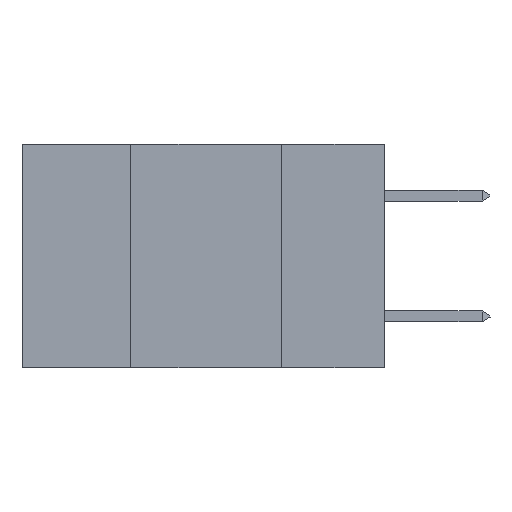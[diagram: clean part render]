
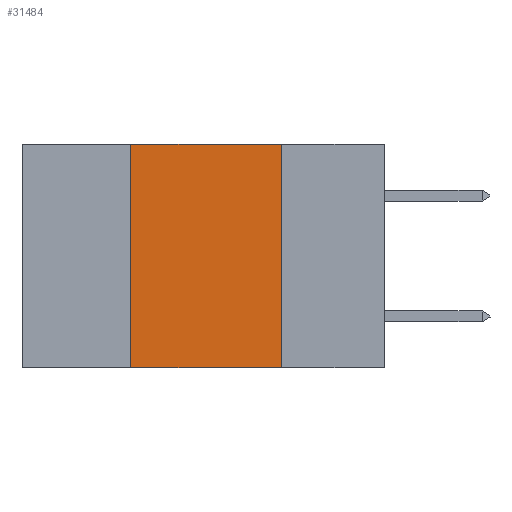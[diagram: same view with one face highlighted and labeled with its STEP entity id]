
A CAD part, left-side view. The second image highlights one B-rep face of the part: STEP entity #31484.
In plain terms, the highlighted planar face has unit normal (-1, 0, 0).
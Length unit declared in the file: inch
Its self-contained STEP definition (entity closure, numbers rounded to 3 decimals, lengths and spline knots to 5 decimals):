
#543 = FACE_OUTER_BOUND ( 'NONE', #5892, .T. ) ;
#1035 = CARTESIAN_POINT ( 'NONE',  ( 0., 0.6, -0.37 ) ) ;
#2490 = CARTESIAN_POINT ( 'NONE',  ( 0., 0.17, -0.37 ) ) ;
#3520 = ORIENTED_EDGE ( 'NONE', *, *, #5733, .F. ) ;
#5733 = EDGE_CURVE ( 'NONE', #18962, #36356, #24256, .T. ) ;
#5892 = EDGE_LOOP ( 'NONE', ( #11558, #26193, #3520, #23856 ) ) ;
#5940 = VECTOR ( 'NONE', #36584, 39.37008 ) ;
#8122 = LINE ( 'NONE', #17236, #39763 ) ;
#10659 = DIRECTION ( 'NONE',  ( 0., -1., 0. ) ) ;
#11173 = LINE ( 'NONE', #16390, #33900 ) ;
#11558 = ORIENTED_EDGE ( 'NONE', *, *, #17591, .F. ) ;
#14889 = DIRECTION ( 'NONE',  ( 1., 0., 0. ) ) ;
#16390 = CARTESIAN_POINT ( 'NONE',  ( 0., 0.17, 0. ) ) ;
#17236 = CARTESIAN_POINT ( 'NONE',  ( 0., 0.6, 0. ) ) ;
#17346 = CARTESIAN_POINT ( 'NONE',  ( 0., 0.42, 0. ) ) ;
#17591 = EDGE_CURVE ( 'NONE', #40217, #25100, #11173, .T. ) ;
#18962 = VERTEX_POINT ( 'NONE', #36440 ) ;
#19039 = CARTESIAN_POINT ( 'NONE',  ( 0., 0.42, 0. ) ) ;
#21131 = PLANE ( 'NONE',  #21215 ) ;
#21215 = AXIS2_PLACEMENT_3D ( 'NONE', #30501, #14889, #23902 ) ;
#23856 = ORIENTED_EDGE ( 'NONE', *, *, #30730, .T. ) ;
#23902 = DIRECTION ( 'NONE',  ( 0., 0., -1. ) ) ;
#24256 = LINE ( 'NONE', #17346, #5940 ) ;
#24322 = LINE ( 'NONE', #1035, #34721 ) ;
#25100 = VERTEX_POINT ( 'NONE', #2490 ) ;
#26193 = ORIENTED_EDGE ( 'NONE', *, *, #35429, .F. ) ;
#26790 = DIRECTION ( 'NONE',  ( 0., -1., 0. ) ) ;
#30501 = CARTESIAN_POINT ( 'NONE',  ( 0., 0.6, 0. ) ) ;
#30730 = EDGE_CURVE ( 'NONE', #18962, #25100, #24322, .T. ) ;
#31469 = CARTESIAN_POINT ( 'NONE',  ( 0., 0.17, 0. ) ) ;
#31484 = ADVANCED_FACE ( 'NONE', ( #543 ), #21131, .F. ) ;
#33900 = VECTOR ( 'NONE', #38380, 39.37008 ) ;
#34721 = VECTOR ( 'NONE', #10659, 39.37008 ) ;
#35429 = EDGE_CURVE ( 'NONE', #36356, #40217, #8122, .T. ) ;
#36356 = VERTEX_POINT ( 'NONE', #19039 ) ;
#36440 = CARTESIAN_POINT ( 'NONE',  ( 0., 0.42, -0.37 ) ) ;
#36584 = DIRECTION ( 'NONE',  ( 0., 0., 1. ) ) ;
#38380 = DIRECTION ( 'NONE',  ( 0., 0., -1. ) ) ;
#39763 = VECTOR ( 'NONE', #26790, 39.37008 ) ;
#40217 = VERTEX_POINT ( 'NONE', #31469 ) ;
